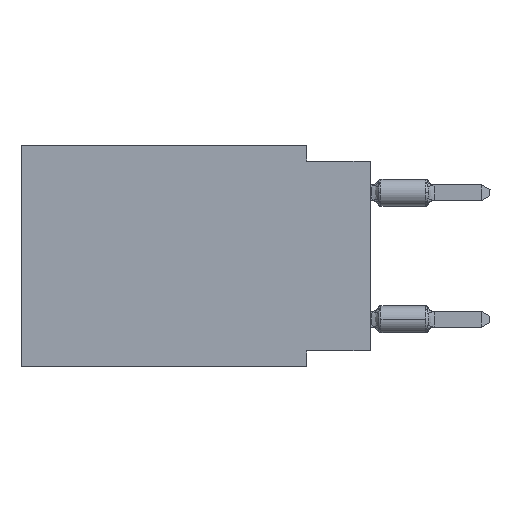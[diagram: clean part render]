
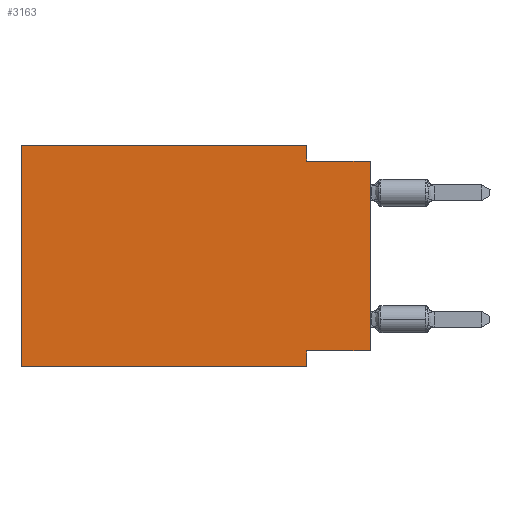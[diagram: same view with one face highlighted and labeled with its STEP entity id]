
A CAD part, left-side view. The second image highlights one B-rep face of the part: STEP entity #3163.
In plain terms, the highlighted planar face has unit normal (-1, 0, 0).
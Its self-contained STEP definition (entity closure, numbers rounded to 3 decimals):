
#28 = ORIENTED_EDGE ( 'NONE', *, *, #2771, .F. ) ;
#144 = VERTEX_POINT ( 'NONE', #719 ) ;
#467 = ORIENTED_EDGE ( 'NONE', *, *, #10985, .T. ) ;
#719 = CARTESIAN_POINT ( 'NONE',  ( 0., 0., -8.255 ) ) ;
#1299 = LINE ( 'NONE', #19491, #3855 ) ;
#1304 = EDGE_CURVE ( 'NONE', #7275, #18018, #12898, .T. ) ;
#1415 = CARTESIAN_POINT ( 'NONE',  ( 0., 2.54, -8.255 ) ) ;
#1534 = LINE ( 'NONE', #8779, #20229 ) ;
#1928 = VERTEX_POINT ( 'NONE', #20963 ) ;
#1955 = VECTOR ( 'NONE', #12268, 1000. ) ;
#2771 = EDGE_CURVE ( 'NONE', #19794, #19488, #21344, .T. ) ;
#2820 = CARTESIAN_POINT ( 'NONE',  ( 0., 2.54, 0. ) ) ;
#3163 = ADVANCED_FACE ( 'NONE', ( #21437 ), #12473, .F. ) ;
#3172 = LINE ( 'NONE', #17397, #1955 ) ;
#3574 = ORIENTED_EDGE ( 'NONE', *, *, #1304, .F. ) ;
#3851 = VERTEX_POINT ( 'NONE', #13585 ) ;
#3855 = VECTOR ( 'NONE', #10637, 1000. ) ;
#4344 = VECTOR ( 'NONE', #10746, 1000. ) ;
#5737 = EDGE_CURVE ( 'NONE', #19488, #3851, #1299, .T. ) ;
#6219 = VECTOR ( 'NONE', #17278, 1000. ) ;
#6761 = CARTESIAN_POINT ( 'NONE',  ( 0., 2.54, -8.89 ) ) ;
#7165 = ORIENTED_EDGE ( 'NONE', *, *, #13601, .F. ) ;
#7275 = VERTEX_POINT ( 'NONE', #18897 ) ;
#7908 = EDGE_CURVE ( 'NONE', #144, #8118, #9402, .T. ) ;
#8118 = VERTEX_POINT ( 'NONE', #1415 ) ;
#8764 = LINE ( 'NONE', #6761, #6219 ) ;
#8779 = CARTESIAN_POINT ( 'NONE',  ( 0., 0., 0. ) ) ;
#8808 = ORIENTED_EDGE ( 'NONE', *, *, #5737, .F. ) ;
#9402 = LINE ( 'NONE', #21767, #16714 ) ;
#10308 = CARTESIAN_POINT ( 'NONE',  ( 0., 2.54, -0.635 ) ) ;
#10637 = DIRECTION ( 'NONE',  ( 0., -1., 0. ) ) ;
#10679 = AXIS2_PLACEMENT_3D ( 'NONE', #12118, #15734, #19683 ) ;
#10746 = DIRECTION ( 'NONE',  ( 0., 0., -1. ) ) ;
#10985 = EDGE_CURVE ( 'NONE', #7275, #1928, #3172, .T. ) ;
#11209 = EDGE_LOOP ( 'NONE', ( #20477, #8808, #28, #7165, #3574, #467, #14611, #20009 ) ) ;
#12118 = CARTESIAN_POINT ( 'NONE',  ( 0., 13.97, 0. ) ) ;
#12131 = DIRECTION ( 'NONE',  ( 0., -1., 0. ) ) ;
#12268 = DIRECTION ( 'NONE',  ( 0., -1., 0. ) ) ;
#12473 = PLANE ( 'NONE',  #10679 ) ;
#12898 = LINE ( 'NONE', #14865, #18976 ) ;
#13256 = DIRECTION ( 'NONE',  ( 0., 1., 0. ) ) ;
#13530 = VECTOR ( 'NONE', #12131, 1000. ) ;
#13585 = CARTESIAN_POINT ( 'NONE',  ( 0., 0., -0.635 ) ) ;
#13601 = EDGE_CURVE ( 'NONE', #18018, #19794, #15511, .T. ) ;
#14472 = CARTESIAN_POINT ( 'NONE',  ( 0., 2.54, 0. ) ) ;
#14611 = ORIENTED_EDGE ( 'NONE', *, *, #19823, .F. ) ;
#14865 = CARTESIAN_POINT ( 'NONE',  ( 0., 13.97, 0. ) ) ;
#15175 = EDGE_CURVE ( 'NONE', #144, #3851, #1534, .T. ) ;
#15511 = LINE ( 'NONE', #19013, #13530 ) ;
#15734 = DIRECTION ( 'NONE',  ( 1., 0., 0. ) ) ;
#16714 = VECTOR ( 'NONE', #13256, 1000. ) ;
#17278 = DIRECTION ( 'NONE',  ( 0., 0., -1. ) ) ;
#17397 = CARTESIAN_POINT ( 'NONE',  ( 0., 13.97, -8.89 ) ) ;
#17647 = DIRECTION ( 'NONE',  ( 0., 0., 1. ) ) ;
#18018 = VERTEX_POINT ( 'NONE', #19045 ) ;
#18897 = CARTESIAN_POINT ( 'NONE',  ( 0., 13.97, -8.89 ) ) ;
#18976 = VECTOR ( 'NONE', #19892, 1000. ) ;
#19013 = CARTESIAN_POINT ( 'NONE',  ( 0., 13.97, 0. ) ) ;
#19045 = CARTESIAN_POINT ( 'NONE',  ( 0., 13.97, 0. ) ) ;
#19488 = VERTEX_POINT ( 'NONE', #10308 ) ;
#19491 = CARTESIAN_POINT ( 'NONE',  ( 0., 0., -0.635 ) ) ;
#19683 = DIRECTION ( 'NONE',  ( 0., 0., -1. ) ) ;
#19794 = VERTEX_POINT ( 'NONE', #2820 ) ;
#19823 = EDGE_CURVE ( 'NONE', #8118, #1928, #8764, .T. ) ;
#19892 = DIRECTION ( 'NONE',  ( 0., 0., 1. ) ) ;
#20009 = ORIENTED_EDGE ( 'NONE', *, *, #7908, .F. ) ;
#20229 = VECTOR ( 'NONE', #17647, 1000. ) ;
#20477 = ORIENTED_EDGE ( 'NONE', *, *, #15175, .T. ) ;
#20963 = CARTESIAN_POINT ( 'NONE',  ( 0., 2.54, -8.89 ) ) ;
#21344 = LINE ( 'NONE', #14472, #4344 ) ;
#21437 = FACE_OUTER_BOUND ( 'NONE', #11209, .T. ) ;
#21767 = CARTESIAN_POINT ( 'NONE',  ( 0., 0., -8.255 ) ) ;
